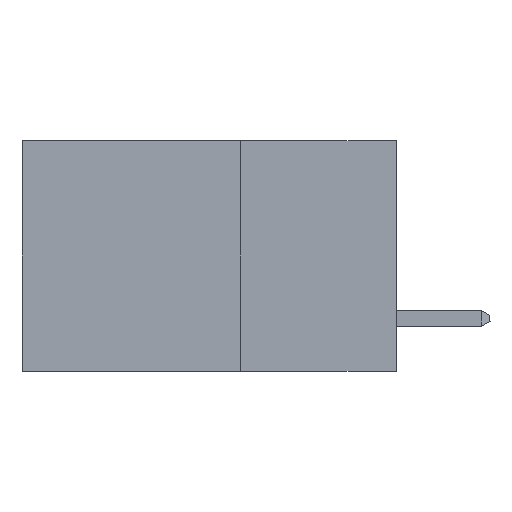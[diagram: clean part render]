
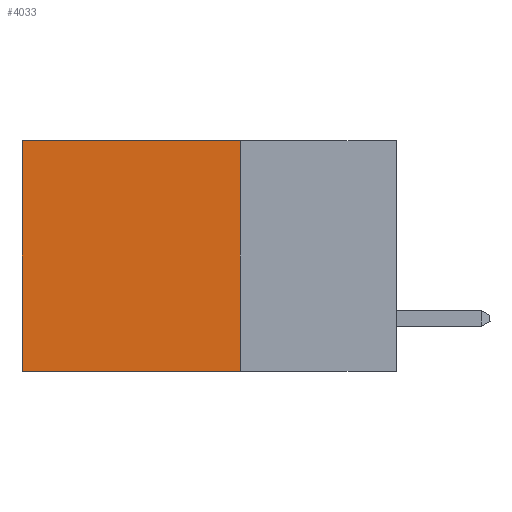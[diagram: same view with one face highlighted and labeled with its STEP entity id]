
A CAD part, left-side view. The second image highlights one B-rep face of the part: STEP entity #4033.
In plain terms, the highlighted planar face has unit normal (-1, 0, 0).
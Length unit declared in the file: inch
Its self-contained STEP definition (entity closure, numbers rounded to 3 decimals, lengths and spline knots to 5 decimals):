
#218 = ORIENTED_EDGE ( 'NONE', *, *, #448, .T. ) ;
#448 = EDGE_CURVE ( 'NONE', #2968, #12772, #9597, .T. ) ;
#691 = LINE ( 'NONE', #3098, #8903 ) ;
#1200 = DIRECTION ( 'NONE',  ( 0., 1., 0. ) ) ;
#1423 = VERTEX_POINT ( 'NONE', #11584 ) ;
#1744 = EDGE_CURVE ( 'NONE', #1423, #11194, #691, .T. ) ;
#2623 = PLANE ( 'NONE',  #8107 ) ;
#2968 = VERTEX_POINT ( 'NONE', #11956 ) ;
#3098 = CARTESIAN_POINT ( 'NONE',  ( 0.298, 0.25, 0. ) ) ;
#3124 = VECTOR ( 'NONE', #5542, 39.37008 ) ;
#3451 = LINE ( 'NONE', #9850, #3124 ) ;
#4033 = ADVANCED_FACE ( 'NONE', ( #11321 ), #2623, .F. ) ;
#4167 = DIRECTION ( 'NONE',  ( 0., 0., -1. ) ) ;
#4864 = ORIENTED_EDGE ( 'NONE', *, *, #13040, .F. ) ;
#5275 = EDGE_LOOP ( 'NONE', ( #218, #4864, #12629, #7363 ) ) ;
#5289 = DIRECTION ( 'NONE',  ( 0., 0., -1. ) ) ;
#5542 = DIRECTION ( 'NONE',  ( 0., 1., 0. ) ) ;
#6637 = DIRECTION ( 'NONE',  ( 0., 0., -1. ) ) ;
#7363 = ORIENTED_EDGE ( 'NONE', *, *, #8374, .T. ) ;
#7461 = VECTOR ( 'NONE', #1200, 39.37008 ) ;
#8107 = AXIS2_PLACEMENT_3D ( 'NONE', #8707, #11933, #6637 ) ;
#8374 = EDGE_CURVE ( 'NONE', #1423, #2968, #3451, .T. ) ;
#8707 = CARTESIAN_POINT ( 'NONE',  ( 0.298, 0.25, 0. ) ) ;
#8903 = VECTOR ( 'NONE', #4167, 39.37008 ) ;
#9237 = CARTESIAN_POINT ( 'NONE',  ( 0.298, 0.6, -0.37 ) ) ;
#9309 = CARTESIAN_POINT ( 'NONE',  ( 0.298, 0.6, 0. ) ) ;
#9597 = LINE ( 'NONE', #9309, #12863 ) ;
#9850 = CARTESIAN_POINT ( 'NONE',  ( 0.298, 0.25, 0. ) ) ;
#11194 = VERTEX_POINT ( 'NONE', #12036 ) ;
#11321 = FACE_OUTER_BOUND ( 'NONE', #5275, .T. ) ;
#11584 = CARTESIAN_POINT ( 'NONE',  ( 0.298, 0.25, 0. ) ) ;
#11933 = DIRECTION ( 'NONE',  ( 1., 0., 0. ) ) ;
#11956 = CARTESIAN_POINT ( 'NONE',  ( 0.298, 0.6, 0. ) ) ;
#12036 = CARTESIAN_POINT ( 'NONE',  ( 0.298, 0.25, -0.37 ) ) ;
#12537 = CARTESIAN_POINT ( 'NONE',  ( 0.298, 0.25, -0.37 ) ) ;
#12629 = ORIENTED_EDGE ( 'NONE', *, *, #1744, .F. ) ;
#12772 = VERTEX_POINT ( 'NONE', #9237 ) ;
#12863 = VECTOR ( 'NONE', #5289, 39.37008 ) ;
#12985 = LINE ( 'NONE', #12537, #7461 ) ;
#13040 = EDGE_CURVE ( 'NONE', #11194, #12772, #12985, .T. ) ;
